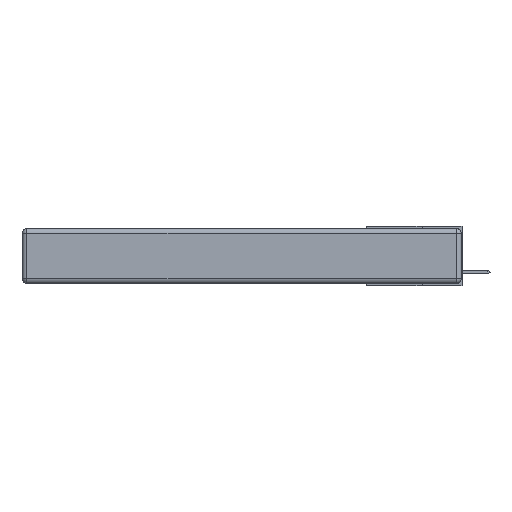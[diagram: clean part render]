
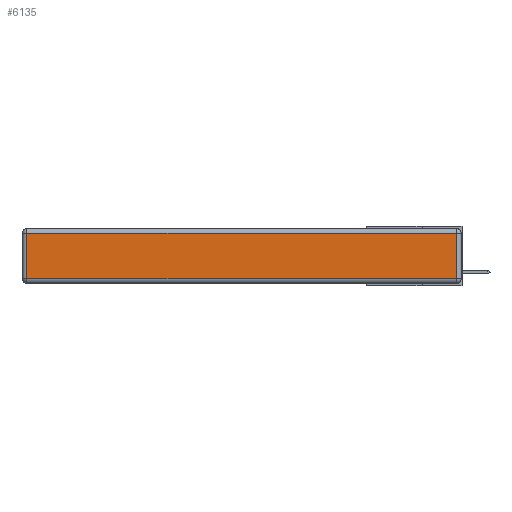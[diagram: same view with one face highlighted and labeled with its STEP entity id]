
A CAD part, left-side view. The second image highlights one B-rep face of the part: STEP entity #6135.
In plain terms, the highlighted planar face has unit normal (-1, 0, 0).
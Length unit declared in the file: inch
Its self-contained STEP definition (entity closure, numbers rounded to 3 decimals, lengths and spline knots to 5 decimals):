
#409 = VECTOR ( 'NONE', #21250, 39.37008 ) ;
#727 = DIRECTION ( 'NONE',  ( 0., 0., -1. ) ) ;
#2614 = ORIENTED_EDGE ( 'NONE', *, *, #11800, .T. ) ;
#3009 = VERTEX_POINT ( 'NONE', #16165 ) ;
#3221 = EDGE_CURVE ( 'NONE', #14290, #3304, #11952, .T. ) ;
#3304 = VERTEX_POINT ( 'NONE', #6190 ) ;
#3367 = VECTOR ( 'NONE', #727, 39.37008 ) ;
#4320 = PLANE ( 'NONE',  #20503 ) ;
#4400 = CARTESIAN_POINT ( 'NONE',  ( 0., 2.72, -0.313 ) ) ;
#5790 = VECTOR ( 'NONE', #11862, 39.37008 ) ;
#6135 = ADVANCED_FACE ( 'NONE', ( #9204 ), #4320, .T. ) ;
#6190 = CARTESIAN_POINT ( 'NONE',  ( 0., 0.03, -0.313 ) ) ;
#8297 = LINE ( 'NONE', #13816, #3367 ) ;
#8316 = CARTESIAN_POINT ( 'NONE',  ( 0., 2.72, -0.03 ) ) ;
#9204 = FACE_OUTER_BOUND ( 'NONE', #15360, .T. ) ;
#9770 = DIRECTION ( 'NONE',  ( 0., 0., 1. ) ) ;
#10376 = EDGE_CURVE ( 'NONE', #3304, #3009, #20044, .T. ) ;
#10527 = EDGE_CURVE ( 'NONE', #3009, #19033, #22092, .T. ) ;
#11800 = EDGE_CURVE ( 'NONE', #19033, #14290, #8297, .T. ) ;
#11862 = DIRECTION ( 'NONE',  ( 0., -1., 0. ) ) ;
#11952 = LINE ( 'NONE', #23101, #5790 ) ;
#12443 = ORIENTED_EDGE ( 'NONE', *, *, #10527, .T. ) ;
#13000 = ORIENTED_EDGE ( 'NONE', *, *, #10376, .T. ) ;
#13816 = CARTESIAN_POINT ( 'NONE',  ( 0., 2.72, -0.343 ) ) ;
#14225 = CARTESIAN_POINT ( 'NONE',  ( 0., 2.75, -0.03 ) ) ;
#14290 = VERTEX_POINT ( 'NONE', #4400 ) ;
#15360 = EDGE_LOOP ( 'NONE', ( #15707, #13000, #12443, #2614 ) ) ;
#15707 = ORIENTED_EDGE ( 'NONE', *, *, #3221, .T. ) ;
#16165 = CARTESIAN_POINT ( 'NONE',  ( 0., 0.03, -0.03 ) ) ;
#17116 = VECTOR ( 'NONE', #23303, 39.37008 ) ;
#19033 = VERTEX_POINT ( 'NONE', #8316 ) ;
#19227 = CARTESIAN_POINT ( 'NONE',  ( 0., 0., -0.343 ) ) ;
#20044 = LINE ( 'NONE', #23075, #409 ) ;
#20503 = AXIS2_PLACEMENT_3D ( 'NONE', #19227, #23002, #9770 ) ;
#21250 = DIRECTION ( 'NONE',  ( 0., 0., 1. ) ) ;
#22092 = LINE ( 'NONE', #14225, #17116 ) ;
#23002 = DIRECTION ( 'NONE',  ( -1., 0., 0. ) ) ;
#23075 = CARTESIAN_POINT ( 'NONE',  ( 0., 0.03, -0.343 ) ) ;
#23101 = CARTESIAN_POINT ( 'NONE',  ( 0., 0., -0.313 ) ) ;
#23303 = DIRECTION ( 'NONE',  ( 0., 1., 0. ) ) ;
